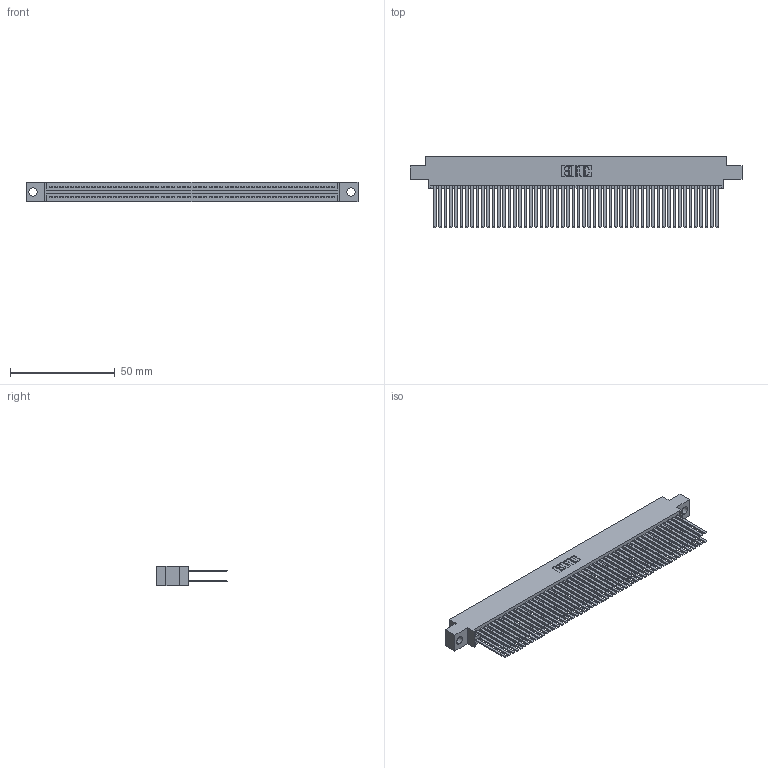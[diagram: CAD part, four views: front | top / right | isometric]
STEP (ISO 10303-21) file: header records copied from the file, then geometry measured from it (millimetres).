
FILE_DESCRIPTION (( 'STEP AP203' ), '1' );
FILE_NAME ('345-108-544-804.STEP', '2018-10-07T07:06:17', ( '' ), ( '' ), 'SwSTEP 2.0', 'SolidWorks 2016', '' );
FILE_SCHEMA (( 'CONFIG_CONTROL_DESIGN' ));
Length unit declared in the file: inch
Products named in the file (3): 345 Part_0.170 Offset - 0.156 Dia-TH; 345-292-001_345-293-144; 345-108-544-804
Assembly tree (109 placements, depth 2):
  345-108-544-804
    345 Part_0.170 Offset - 0.156 Dia-TH
    345-292-001_345-293-144  x108
Bounding box: 158.37 x 33.96 x 9.4 mm (x, y, z)
Volume: 16808.2 mm3; surface area: 29473.7 mm2
Topology: 109 solids, 109 shells, 4882 faces, 14501 edges, 9522 vertices
Faces by surface type: plane 3216, cylinder 1666
Entity records: 40705 total; most frequent: CARTESIAN_POINT 6812, ORIENTED_EDGE 6746, DIRECTION 5989, EDGE_CURVE 3373, VECTOR 3029, LINE 3029, VERTEX_POINT 2246, AXIS2_PLACEMENT_3D 1480
